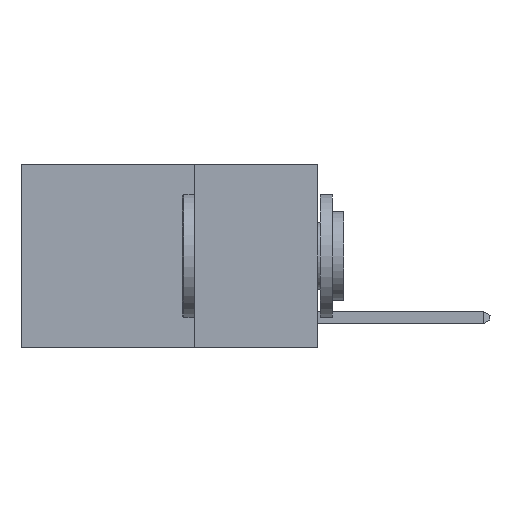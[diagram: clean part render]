
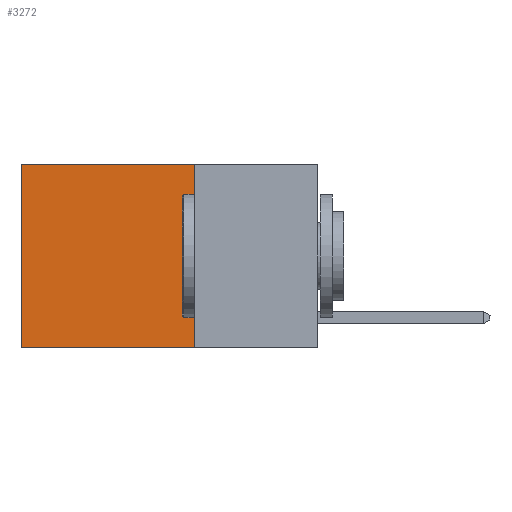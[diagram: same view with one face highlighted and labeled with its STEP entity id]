
A CAD part, left-side view. The second image highlights one B-rep face of the part: STEP entity #3272.
In plain terms, the highlighted planar face has unit normal (-1, 0, 0).
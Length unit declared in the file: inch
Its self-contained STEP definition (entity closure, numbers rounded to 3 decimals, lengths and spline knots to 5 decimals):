
#493 = VERTEX_POINT ( 'NONE', #11996 ) ;
#862 = VECTOR ( 'NONE', #2524, 39.37008 ) ;
#1259 = CARTESIAN_POINT ( 'NONE',  ( 0.2625, 0.6, -0.37 ) ) ;
#1289 = DIRECTION ( 'NONE',  ( 0., 0., -1. ) ) ;
#1547 = CARTESIAN_POINT ( 'NONE',  ( 0.2625, 0.25, 0. ) ) ;
#1956 = ORIENTED_EDGE ( 'NONE', *, *, #7475, .F. ) ;
#2291 = PLANE ( 'NONE',  #10316 ) ;
#2503 = LINE ( 'NONE', #3507, #7421 ) ;
#2524 = DIRECTION ( 'NONE',  ( 0., 1., 0. ) ) ;
#3260 = LINE ( 'NONE', #5198, #7859 ) ;
#3272 = ADVANCED_FACE ( 'NONE', ( #12384 ), #2291, .F. ) ;
#3451 = VECTOR ( 'NONE', #6064, 39.37008 ) ;
#3507 = CARTESIAN_POINT ( 'NONE',  ( 0.2625, 0.25, -0.37 ) ) ;
#4272 = DIRECTION ( 'NONE',  ( 1., 0., 0. ) ) ;
#4609 = EDGE_LOOP ( 'NONE', ( #6557, #12052, #1956, #12355 ) ) ;
#5198 = CARTESIAN_POINT ( 'NONE',  ( 0.2625, 0.25, 0. ) ) ;
#6016 = CARTESIAN_POINT ( 'NONE',  ( 0.2625, 0.6, 0. ) ) ;
#6064 = DIRECTION ( 'NONE',  ( 0., 0., -1. ) ) ;
#6387 = EDGE_CURVE ( 'NONE', #10749, #12185, #2503, .T. ) ;
#6557 = ORIENTED_EDGE ( 'NONE', *, *, #10009, .T. ) ;
#7269 = VERTEX_POINT ( 'NONE', #10727 ) ;
#7421 = VECTOR ( 'NONE', #11337, 39.37008 ) ;
#7475 = EDGE_CURVE ( 'NONE', #7269, #10749, #3260, .T. ) ;
#7859 = VECTOR ( 'NONE', #1289, 39.37008 ) ;
#8362 = LINE ( 'NONE', #6016, #3451 ) ;
#8686 = LINE ( 'NONE', #1547, #862 ) ;
#9178 = CARTESIAN_POINT ( 'NONE',  ( 0.2625, 0.25, 0. ) ) ;
#9632 = EDGE_CURVE ( 'NONE', #7269, #493, #8686, .T. ) ;
#9665 = CARTESIAN_POINT ( 'NONE',  ( 0.2625, 0.25, -0.37 ) ) ;
#10009 = EDGE_CURVE ( 'NONE', #493, #12185, #8362, .T. ) ;
#10316 = AXIS2_PLACEMENT_3D ( 'NONE', #9178, #4272, #11119 ) ;
#10727 = CARTESIAN_POINT ( 'NONE',  ( 0.2625, 0.25, 0. ) ) ;
#10749 = VERTEX_POINT ( 'NONE', #9665 ) ;
#11119 = DIRECTION ( 'NONE',  ( 0., 0., -1. ) ) ;
#11337 = DIRECTION ( 'NONE',  ( 0., 1., 0. ) ) ;
#11996 = CARTESIAN_POINT ( 'NONE',  ( 0.2625, 0.6, 0. ) ) ;
#12052 = ORIENTED_EDGE ( 'NONE', *, *, #6387, .F. ) ;
#12185 = VERTEX_POINT ( 'NONE', #1259 ) ;
#12355 = ORIENTED_EDGE ( 'NONE', *, *, #9632, .T. ) ;
#12384 = FACE_OUTER_BOUND ( 'NONE', #4609, .T. ) ;
